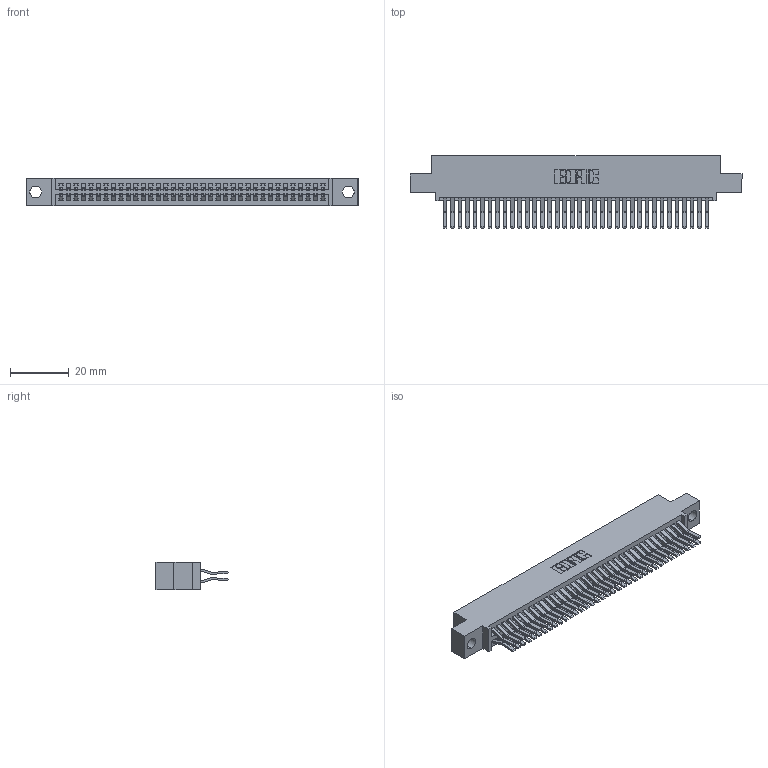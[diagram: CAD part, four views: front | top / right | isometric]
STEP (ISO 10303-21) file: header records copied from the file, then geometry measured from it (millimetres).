
FILE_DESCRIPTION (( 'STEP AP203' ), '1' );
FILE_NAME ('395-072-560-504.STEP', '2021-06-17T05:16:36', ( '' ), ( '' ), 'SwSTEP 2.0', 'SolidWorks 2020', '' );
FILE_SCHEMA (( 'CONFIG_CONTROL_DESIGN' ));
Length unit declared in the file: inch
Products named in the file (3): 395-072-560-504; 345 Part_0.110 Offset - 0.156 Dia-TI; 345-292-001_560 Tail
Assembly tree (73 placements, depth 2):
  395-072-560-504
    345 Part_0.110 Offset - 0.156 Dia-TI
    345-292-001_560 Tail  x72
Bounding box: 112.65 x 24.45 x 9.4 mm (x, y, z)
Volume: 11179.8 mm3; surface area: 17567.5 mm2
Topology: 73 solids, 73 shells, 3888 faces, 11549 edges, 7602 vertices
Faces by surface type: plane 2474, cylinder 1414
Entity records: 29693 total; most frequent: CARTESIAN_POINT 4990, ORIENTED_EDGE 4922, DIRECTION 4409, EDGE_CURVE 2461, VECTOR 2181, LINE 2181, VERTEX_POINT 1638, AXIS2_PLACEMENT_3D 1114
